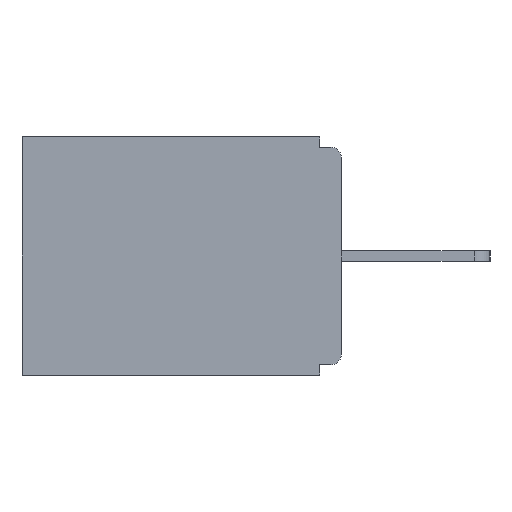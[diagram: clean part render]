
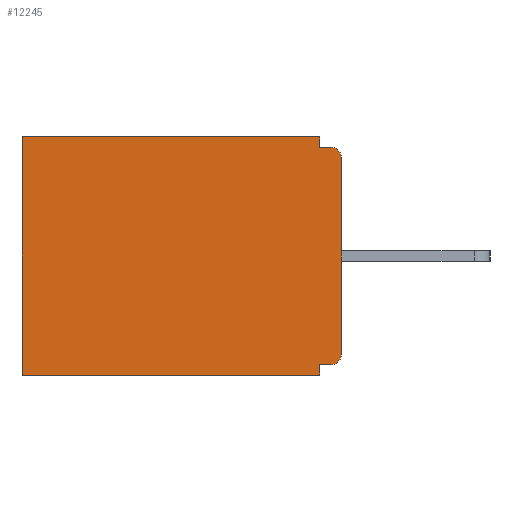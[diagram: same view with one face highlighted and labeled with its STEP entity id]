
A CAD part, left-side view. The second image highlights one B-rep face of the part: STEP entity #12245.
In plain terms, the highlighted planar face has unit normal (-1, 0, 0).
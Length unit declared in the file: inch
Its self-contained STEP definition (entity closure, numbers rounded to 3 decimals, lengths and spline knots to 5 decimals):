
#346 = EDGE_CURVE ( 'NONE', #7896, #12543, #5356, .T. ) ;
#353 = ORIENTED_EDGE ( 'NONE', *, *, #3616, .F. ) ;
#589 = VERTEX_POINT ( 'NONE', #8321 ) ;
#976 = ORIENTED_EDGE ( 'NONE', *, *, #9060, .F. ) ;
#991 = DIRECTION ( 'NONE',  ( 1., 0., 0. ) ) ;
#1474 = DIRECTION ( 'NONE',  ( 0., 1., 0. ) ) ;
#1791 = ORIENTED_EDGE ( 'NONE', *, *, #8397, .F. ) ;
#2039 = CARTESIAN_POINT ( 'NONE',  ( 0.298, 0.015, -0.03 ) ) ;
#2169 = ORIENTED_EDGE ( 'NONE', *, *, #7909, .T. ) ;
#2173 = CIRCLE ( 'NONE', #8422, 0.015 ) ;
#2364 = DIRECTION ( 'NONE',  ( 0., 0., -1. ) ) ;
#2580 = ORIENTED_EDGE ( 'NONE', *, *, #346, .T. ) ;
#2647 = CARTESIAN_POINT ( 'NONE',  ( 0.298, 0.031, 0. ) ) ;
#2973 = CARTESIAN_POINT ( 'NONE',  ( 0.298, 0.031, -0.343 ) ) ;
#3218 = DIRECTION ( 'NONE',  ( -1., 0., 0. ) ) ;
#3616 = EDGE_CURVE ( 'NONE', #11203, #6297, #5963, .T. ) ;
#3920 = LINE ( 'NONE', #5175, #11619 ) ;
#3976 = CARTESIAN_POINT ( 'NONE',  ( 0.298, 0.46, 0. ) ) ;
#4357 = DIRECTION ( 'NONE',  ( 0., 0., -1. ) ) ;
#4501 = CARTESIAN_POINT ( 'NONE',  ( 0.298, 0.46, 0. ) ) ;
#4577 = VERTEX_POINT ( 'NONE', #10712 ) ;
#4655 = VERTEX_POINT ( 'NONE', #8567 ) ;
#5175 = CARTESIAN_POINT ( 'NONE',  ( 0.298, 0., -0.343 ) ) ;
#5347 = EDGE_CURVE ( 'NONE', #11203, #589, #8390, .T. ) ;
#5356 = LINE ( 'NONE', #11394, #5442 ) ;
#5442 = VECTOR ( 'NONE', #8813, 39.37008 ) ;
#5597 = CARTESIAN_POINT ( 'NONE',  ( 0.298, 0., -0.313 ) ) ;
#5802 = CARTESIAN_POINT ( 'NONE',  ( 0.298, 0., 0. ) ) ;
#5963 = LINE ( 'NONE', #5802, #6572 ) ;
#6297 = VERTEX_POINT ( 'NONE', #5597 ) ;
#6572 = VECTOR ( 'NONE', #15493, 39.37008 ) ;
#6654 = DIRECTION ( 'NONE',  ( 0., 0., -1. ) ) ;
#6673 = CARTESIAN_POINT ( 'NONE',  ( 0.298, 0.015, -0.328 ) ) ;
#6698 = CARTESIAN_POINT ( 'NONE',  ( 0.298, 0., -0.015 ) ) ;
#6865 = EDGE_CURVE ( 'NONE', #7013, #6297, #2173, .T. ) ;
#7013 = VERTEX_POINT ( 'NONE', #6673 ) ;
#7037 = FACE_OUTER_BOUND ( 'NONE', #11805, .T. ) ;
#7112 = CARTESIAN_POINT ( 'NONE',  ( 0.298, 0., 0. ) ) ;
#7352 = LINE ( 'NONE', #9640, #8989 ) ;
#7474 = CARTESIAN_POINT ( 'NONE',  ( 0.298, 0.46, -0.343 ) ) ;
#7636 = CARTESIAN_POINT ( 'NONE',  ( 0.298, 0., -0.03 ) ) ;
#7710 = ORIENTED_EDGE ( 'NONE', *, *, #13192, .F. ) ;
#7896 = VERTEX_POINT ( 'NONE', #2647 ) ;
#7909 = EDGE_CURVE ( 'NONE', #12543, #14266, #9961, .T. ) ;
#7991 = VECTOR ( 'NONE', #13853, 39.37008 ) ;
#8321 = CARTESIAN_POINT ( 'NONE',  ( 0.298, 0.015, -0.015 ) ) ;
#8390 = CIRCLE ( 'NONE', #12646, 0.015 ) ;
#8397 = EDGE_CURVE ( 'NONE', #7896, #4655, #11541, .T. ) ;
#8422 = AXIS2_PLACEMENT_3D ( 'NONE', #9312, #14195, #4357 ) ;
#8541 = DIRECTION ( 'NONE',  ( 0., 1., 0. ) ) ;
#8567 = CARTESIAN_POINT ( 'NONE',  ( 0.298, 0.031, -0.015 ) ) ;
#8764 = DIRECTION ( 'NONE',  ( 0., 0., -1. ) ) ;
#8813 = DIRECTION ( 'NONE',  ( 0., 1., 0. ) ) ;
#8943 = LINE ( 'NONE', #2973, #10140 ) ;
#8989 = VECTOR ( 'NONE', #1474, 39.37008 ) ;
#9060 = EDGE_CURVE ( 'NONE', #7013, #4577, #7352, .T. ) ;
#9312 = CARTESIAN_POINT ( 'NONE',  ( 0.298, 0.015, -0.313 ) ) ;
#9640 = CARTESIAN_POINT ( 'NONE',  ( 0.298, 0., -0.328 ) ) ;
#9715 = EDGE_CURVE ( 'NONE', #4655, #589, #11558, .T. ) ;
#9961 = LINE ( 'NONE', #3976, #11470 ) ;
#10140 = VECTOR ( 'NONE', #6654, 39.37008 ) ;
#10503 = DIRECTION ( 'NONE',  ( 0., 0., -1. ) ) ;
#10712 = CARTESIAN_POINT ( 'NONE',  ( 0.298, 0.031, -0.328 ) ) ;
#11203 = VERTEX_POINT ( 'NONE', #7636 ) ;
#11394 = CARTESIAN_POINT ( 'NONE',  ( 0.298, 0., 0. ) ) ;
#11470 = VECTOR ( 'NONE', #8764, 39.37008 ) ;
#11541 = LINE ( 'NONE', #13033, #14498 ) ;
#11558 = LINE ( 'NONE', #6698, #7991 ) ;
#11619 = VECTOR ( 'NONE', #8541, 39.37008 ) ;
#11743 = PLANE ( 'NONE',  #13627 ) ;
#11805 = EDGE_LOOP ( 'NONE', ( #13025, #15477, #1791, #2580, #2169, #13746, #7710, #976, #13953, #353 ) ) ;
#12245 = ADVANCED_FACE ( 'NONE', ( #7037 ), #11743, .F. ) ;
#12543 = VERTEX_POINT ( 'NONE', #4501 ) ;
#12646 = AXIS2_PLACEMENT_3D ( 'NONE', #2039, #3218, #14062 ) ;
#13025 = ORIENTED_EDGE ( 'NONE', *, *, #5347, .T. ) ;
#13033 = CARTESIAN_POINT ( 'NONE',  ( 0.298, 0.031, -0.343 ) ) ;
#13040 = VERTEX_POINT ( 'NONE', #15568 ) ;
#13046 = EDGE_CURVE ( 'NONE', #13040, #14266, #3920, .T. ) ;
#13192 = EDGE_CURVE ( 'NONE', #4577, #13040, #8943, .T. ) ;
#13627 = AXIS2_PLACEMENT_3D ( 'NONE', #7112, #991, #10503 ) ;
#13746 = ORIENTED_EDGE ( 'NONE', *, *, #13046, .F. ) ;
#13853 = DIRECTION ( 'NONE',  ( 0., -1., 0. ) ) ;
#13953 = ORIENTED_EDGE ( 'NONE', *, *, #6865, .T. ) ;
#14062 = DIRECTION ( 'NONE',  ( 0., 0., -1. ) ) ;
#14195 = DIRECTION ( 'NONE',  ( -1., 0., 0. ) ) ;
#14266 = VERTEX_POINT ( 'NONE', #7474 ) ;
#14498 = VECTOR ( 'NONE', #2364, 39.37008 ) ;
#15477 = ORIENTED_EDGE ( 'NONE', *, *, #9715, .F. ) ;
#15493 = DIRECTION ( 'NONE',  ( 0., 0., -1. ) ) ;
#15568 = CARTESIAN_POINT ( 'NONE',  ( 0.298, 0.031, -0.343 ) ) ;
